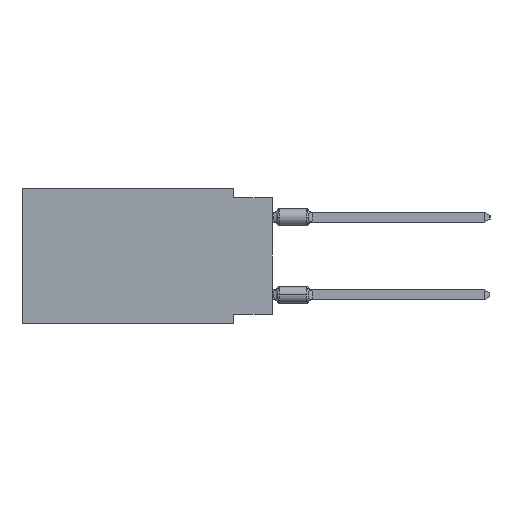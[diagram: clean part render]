
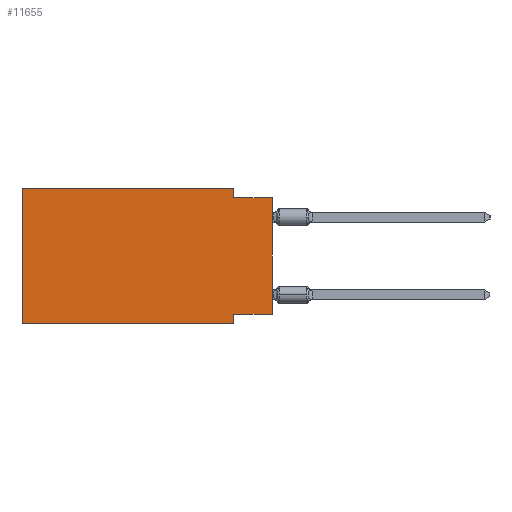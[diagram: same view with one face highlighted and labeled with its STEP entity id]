
A CAD part, left-side view. The second image highlights one B-rep face of the part: STEP entity #11655.
In plain terms, the highlighted planar face has unit normal (-1, 0, 0).
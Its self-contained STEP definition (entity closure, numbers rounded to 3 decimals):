
#1452 = ORIENTED_EDGE ( 'NONE', *, *, #13334, .F. ) ;
#1997 = VERTEX_POINT ( 'NONE', #35155 ) ;
#2031 = LINE ( 'NONE', #6460, #16180 ) ;
#2592 = DIRECTION ( 'NONE',  ( 0., 0., 1. ) ) ;
#2977 = DIRECTION ( 'NONE',  ( 0., 1., 0. ) ) ;
#6429 = AXIS2_PLACEMENT_3D ( 'NONE', #31491, #35641, #31239 ) ;
#6460 = CARTESIAN_POINT ( 'NONE',  ( 0., 0., 0. ) ) ;
#7699 = VECTOR ( 'NONE', #2592, 1000. ) ;
#7709 = DIRECTION ( 'NONE',  ( 0., 0., -1. ) ) ;
#8393 = VECTOR ( 'NONE', #43135, 1000. ) ;
#8527 = EDGE_CURVE ( 'NONE', #39174, #17768, #35645, .T. ) ;
#9331 = CARTESIAN_POINT ( 'NONE',  ( 0., 2.54, -8.255 ) ) ;
#10063 = ORIENTED_EDGE ( 'NONE', *, *, #20218, .F. ) ;
#10092 = ORIENTED_EDGE ( 'NONE', *, *, #37991, .F. ) ;
#11250 = CARTESIAN_POINT ( 'NONE',  ( 0., 0., -8.255 ) ) ;
#11368 = LINE ( 'NONE', #43384, #8393 ) ;
#11655 = ADVANCED_FACE ( 'NONE', ( #27846 ), #43200, .F. ) ;
#13121 = ORIENTED_EDGE ( 'NONE', *, *, #43819, .F. ) ;
#13334 = EDGE_CURVE ( 'NONE', #30957, #39174, #11368, .T. ) ;
#14243 = VECTOR ( 'NONE', #2977, 1000. ) ;
#15560 = LINE ( 'NONE', #46790, #42599 ) ;
#15631 = CARTESIAN_POINT ( 'NONE',  ( 0., 16.383, -8.89 ) ) ;
#16180 = VECTOR ( 'NONE', #42147, 1000. ) ;
#16195 = VECTOR ( 'NONE', #45324, 1000. ) ;
#17768 = VERTEX_POINT ( 'NONE', #21904 ) ;
#18004 = CARTESIAN_POINT ( 'NONE',  ( 0., 2.54, -0.635 ) ) ;
#18178 = VECTOR ( 'NONE', #51503, 1000. ) ;
#19035 = LINE ( 'NONE', #15631, #35599 ) ;
#20218 = EDGE_CURVE ( 'NONE', #41135, #30957, #35596, .T. ) ;
#21170 = VERTEX_POINT ( 'NONE', #9331 ) ;
#21904 = CARTESIAN_POINT ( 'NONE',  ( 0., 0., -0.635 ) ) ;
#23941 = CARTESIAN_POINT ( 'NONE',  ( 0., 0., -0.635 ) ) ;
#25881 = ORIENTED_EDGE ( 'NONE', *, *, #8527, .F. ) ;
#26495 = EDGE_CURVE ( 'NONE', #44105, #1997, #19035, .T. ) ;
#27846 = FACE_OUTER_BOUND ( 'NONE', #42149, .T. ) ;
#28305 = VERTEX_POINT ( 'NONE', #11250 ) ;
#29578 = EDGE_CURVE ( 'NONE', #28305, #21170, #33736, .T. ) ;
#30957 = VERTEX_POINT ( 'NONE', #31901 ) ;
#31239 = DIRECTION ( 'NONE',  ( 0., 0., -1. ) ) ;
#31491 = CARTESIAN_POINT ( 'NONE',  ( 0., 16.383, 0. ) ) ;
#31901 = CARTESIAN_POINT ( 'NONE',  ( 0., 2.54, 0. ) ) ;
#33736 = LINE ( 'NONE', #37893, #14243 ) ;
#34122 = LINE ( 'NONE', #50014, #7699 ) ;
#35155 = CARTESIAN_POINT ( 'NONE',  ( 0., 2.54, -8.89 ) ) ;
#35596 = LINE ( 'NONE', #40271, #18178 ) ;
#35599 = VECTOR ( 'NONE', #46870, 1000. ) ;
#35641 = DIRECTION ( 'NONE',  ( 1., 0., 0. ) ) ;
#35645 = LINE ( 'NONE', #23941, #16195 ) ;
#37893 = CARTESIAN_POINT ( 'NONE',  ( 0., 0., -8.255 ) ) ;
#37991 = EDGE_CURVE ( 'NONE', #44105, #41135, #34122, .T. ) ;
#38455 = ORIENTED_EDGE ( 'NONE', *, *, #26495, .T. ) ;
#39174 = VERTEX_POINT ( 'NONE', #18004 ) ;
#39566 = EDGE_CURVE ( 'NONE', #28305, #17768, #2031, .T. ) ;
#40271 = CARTESIAN_POINT ( 'NONE',  ( 0., 16.383, 0. ) ) ;
#41135 = VERTEX_POINT ( 'NONE', #41315 ) ;
#41315 = CARTESIAN_POINT ( 'NONE',  ( 0., 16.383, 0. ) ) ;
#42147 = DIRECTION ( 'NONE',  ( 0., 0., 1. ) ) ;
#42149 = EDGE_LOOP ( 'NONE', ( #48375, #25881, #1452, #10063, #10092, #38455, #13121, #49326 ) ) ;
#42599 = VECTOR ( 'NONE', #7709, 1000. ) ;
#43135 = DIRECTION ( 'NONE',  ( 0., 0., -1. ) ) ;
#43200 = PLANE ( 'NONE',  #6429 ) ;
#43384 = CARTESIAN_POINT ( 'NONE',  ( 0., 2.54, 0. ) ) ;
#43819 = EDGE_CURVE ( 'NONE', #21170, #1997, #15560, .T. ) ;
#44105 = VERTEX_POINT ( 'NONE', #45921 ) ;
#45324 = DIRECTION ( 'NONE',  ( 0., -1., 0. ) ) ;
#45921 = CARTESIAN_POINT ( 'NONE',  ( 0., 16.383, -8.89 ) ) ;
#46790 = CARTESIAN_POINT ( 'NONE',  ( 0., 2.54, -8.89 ) ) ;
#46870 = DIRECTION ( 'NONE',  ( 0., -1., 0. ) ) ;
#48375 = ORIENTED_EDGE ( 'NONE', *, *, #39566, .T. ) ;
#49326 = ORIENTED_EDGE ( 'NONE', *, *, #29578, .F. ) ;
#50014 = CARTESIAN_POINT ( 'NONE',  ( 0., 16.383, 0. ) ) ;
#51503 = DIRECTION ( 'NONE',  ( 0., -1., 0. ) ) ;
